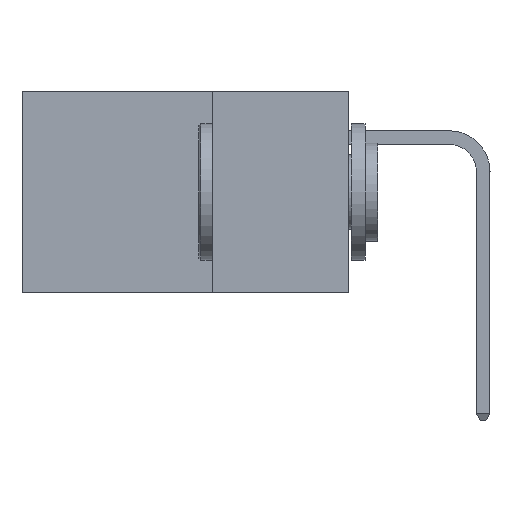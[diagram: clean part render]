
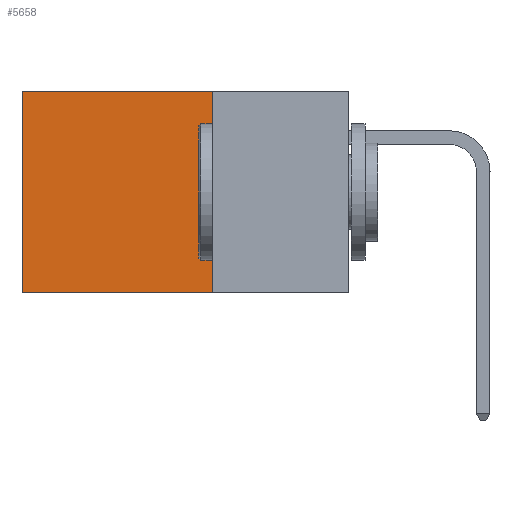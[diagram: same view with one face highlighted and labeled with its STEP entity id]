
A CAD part, left-side view. The second image highlights one B-rep face of the part: STEP entity #5658.
In plain terms, the highlighted planar face has unit normal (-1, 0, 0).
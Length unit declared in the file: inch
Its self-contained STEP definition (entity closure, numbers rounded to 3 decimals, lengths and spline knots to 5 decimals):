
#30 = EDGE_CURVE ( 'NONE', #4974, #5925, #1974, .T. ) ;
#236 = VECTOR ( 'NONE', #6353, 39.37008 ) ;
#272 = DIRECTION ( 'NONE',  ( 1., 0., 0. ) ) ;
#291 = VERTEX_POINT ( 'NONE', #10869 ) ;
#788 = DIRECTION ( 'NONE',  ( 0., 1., 0. ) ) ;
#1106 = CARTESIAN_POINT ( 'NONE',  ( 0.2875, 0.25, 0. ) ) ;
#1966 = DIRECTION ( 'NONE',  ( 0., 0., -1. ) ) ;
#1974 = LINE ( 'NONE', #7163, #236 ) ;
#2094 = ORIENTED_EDGE ( 'NONE', *, *, #7912, .T. ) ;
#2629 = CARTESIAN_POINT ( 'NONE',  ( 0.2875, 0.6, -0.37 ) ) ;
#4368 = LINE ( 'NONE', #11804, #9187 ) ;
#4672 = CARTESIAN_POINT ( 'NONE',  ( 0.2875, 0.25, 0. ) ) ;
#4974 = VERTEX_POINT ( 'NONE', #1106 ) ;
#5524 = FACE_OUTER_BOUND ( 'NONE', #7611, .T. ) ;
#5658 = ADVANCED_FACE ( 'NONE', ( #5524 ), #11463, .F. ) ;
#5925 = VERTEX_POINT ( 'NONE', #11677 ) ;
#6353 = DIRECTION ( 'NONE',  ( 0., 1., 0. ) ) ;
#6801 = AXIS2_PLACEMENT_3D ( 'NONE', #4672, #272, #7570 ) ;
#6977 = LINE ( 'NONE', #11761, #10971 ) ;
#7163 = CARTESIAN_POINT ( 'NONE',  ( 0.2875, 0.25, 0. ) ) ;
#7171 = DIRECTION ( 'NONE',  ( 0., 0., -1. ) ) ;
#7337 = VECTOR ( 'NONE', #1966, 39.37008 ) ;
#7570 = DIRECTION ( 'NONE',  ( 0., 0., -1. ) ) ;
#7611 = EDGE_LOOP ( 'NONE', ( #2094, #7702, #7960, #8227 ) ) ;
#7702 = ORIENTED_EDGE ( 'NONE', *, *, #8516, .F. ) ;
#7912 = EDGE_CURVE ( 'NONE', #5925, #10656, #4368, .T. ) ;
#7960 = ORIENTED_EDGE ( 'NONE', *, *, #10900, .F. ) ;
#7996 = CARTESIAN_POINT ( 'NONE',  ( 0.2875, 0.25, 0. ) ) ;
#8227 = ORIENTED_EDGE ( 'NONE', *, *, #30, .T. ) ;
#8516 = EDGE_CURVE ( 'NONE', #291, #10656, #6977, .T. ) ;
#9187 = VECTOR ( 'NONE', #7171, 39.37008 ) ;
#9217 = LINE ( 'NONE', #7996, #7337 ) ;
#10656 = VERTEX_POINT ( 'NONE', #2629 ) ;
#10869 = CARTESIAN_POINT ( 'NONE',  ( 0.2875, 0.25, -0.37 ) ) ;
#10900 = EDGE_CURVE ( 'NONE', #4974, #291, #9217, .T. ) ;
#10971 = VECTOR ( 'NONE', #788, 39.37008 ) ;
#11463 = PLANE ( 'NONE',  #6801 ) ;
#11677 = CARTESIAN_POINT ( 'NONE',  ( 0.2875, 0.6, 0. ) ) ;
#11761 = CARTESIAN_POINT ( 'NONE',  ( 0.2875, 0.25, -0.37 ) ) ;
#11804 = CARTESIAN_POINT ( 'NONE',  ( 0.2875, 0.6, 0. ) ) ;
